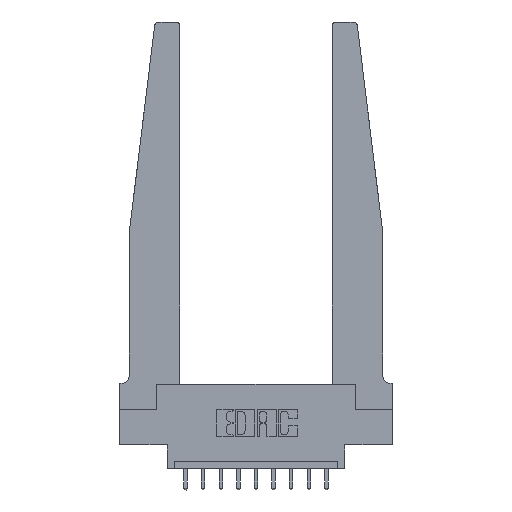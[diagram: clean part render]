
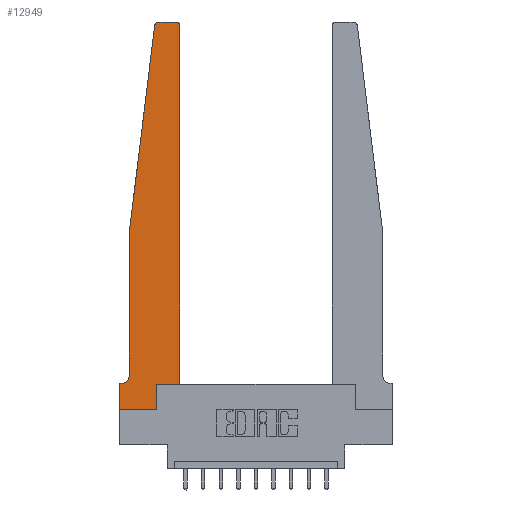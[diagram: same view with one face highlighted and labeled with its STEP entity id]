
A CAD part, top view. The second image highlights one B-rep face of the part: STEP entity #12949.
In plain terms, the highlighted planar face has unit normal (0, 0, 1).
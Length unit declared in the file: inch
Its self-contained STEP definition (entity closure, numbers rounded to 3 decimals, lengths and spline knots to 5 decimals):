
#43 = CARTESIAN_POINT ( 'NONE',  ( 0.065, 0.2375, 0.37 ) ) ;
#141 = EDGE_CURVE ( 'NONE', #6398, #14624, #8336, .T. ) ;
#646 = ORIENTED_EDGE ( 'NONE', *, *, #3364, .T. ) ;
#831 = EDGE_CURVE ( 'NONE', #3341, #6398, #3662, .T. ) ;
#875 = EDGE_CURVE ( 'NONE', #2817, #8710, #5645, .T. ) ;
#887 = LINE ( 'NONE', #10815, #14583 ) ;
#920 = DIRECTION ( 'NONE',  ( 0., -1., 0. ) ) ;
#983 = DIRECTION ( 'NONE',  ( 0., 0., 1. ) ) ;
#1242 = LINE ( 'NONE', #5475, #10400 ) ;
#1786 = DIRECTION ( 'NONE',  ( -0.122, -0.992, 0. ) ) ;
#2125 = VERTEX_POINT ( 'NONE', #9649 ) ;
#2160 = CARTESIAN_POINT ( 'NONE',  ( 0.425, 0.18, 0.37 ) ) ;
#2197 = VERTEX_POINT ( 'NONE', #4325 ) ;
#2322 = DIRECTION ( 'NONE',  ( -1., 0., 0. ) ) ;
#2430 = CARTESIAN_POINT ( 'NONE',  ( 0., 0.1875, 0.37 ) ) ;
#2730 = AXIS2_PLACEMENT_3D ( 'NONE', #3219, #983, #9914 ) ;
#2782 = CARTESIAN_POINT ( 'NONE',  ( 0.395, 2.75, 0.37 ) ) ;
#2817 = VERTEX_POINT ( 'NONE', #5413 ) ;
#3219 = CARTESIAN_POINT ( 'NONE',  ( 0.395, 2.72, 0.37 ) ) ;
#3260 = CARTESIAN_POINT ( 'NONE',  ( 0.065, 1.25, 0.37 ) ) ;
#3332 = VECTOR ( 'NONE', #11493, 39.37008 ) ;
#3341 = VERTEX_POINT ( 'NONE', #3260 ) ;
#3364 = EDGE_CURVE ( 'NONE', #8710, #3982, #12868, .T. ) ;
#3376 = ORIENTED_EDGE ( 'NONE', *, *, #875, .T. ) ;
#3406 = ORIENTED_EDGE ( 'NONE', *, *, #7383, .T. ) ;
#3469 = DIRECTION ( 'NONE',  ( 0., 1., 0. ) ) ;
#3493 = CARTESIAN_POINT ( 'NONE',  ( 0.2605, 0.18, 0.37 ) ) ;
#3662 = LINE ( 'NONE', #11194, #6195 ) ;
#3982 = VERTEX_POINT ( 'NONE', #4528 ) ;
#4040 = AXIS2_PLACEMENT_3D ( 'NONE', #13748, #14932, #2322 ) ;
#4051 = EDGE_CURVE ( 'NONE', #7455, #9309, #7421, .T. ) ;
#4325 = CARTESIAN_POINT ( 'NONE',  ( 0.425, 0.18, 0.37 ) ) ;
#4417 = PLANE ( 'NONE',  #6446 ) ;
#4528 = CARTESIAN_POINT ( 'NONE',  ( 0.27653, 2.75, 0.37 ) ) ;
#4872 = CARTESIAN_POINT ( 'NONE',  ( 0., 0., 0.37 ) ) ;
#4905 = DIRECTION ( 'NONE',  ( 1., 0., 0. ) ) ;
#5065 = LINE ( 'NONE', #2160, #12078 ) ;
#5413 = CARTESIAN_POINT ( 'NONE',  ( 0.425, 2.72, 0.37 ) ) ;
#5475 = CARTESIAN_POINT ( 'NONE',  ( 0., 0., 0.37 ) ) ;
#5494 = DIRECTION ( 'NONE',  ( -1., 0., 0. ) ) ;
#5553 = CARTESIAN_POINT ( 'NONE',  ( 0.425, 0.18, 0.37 ) ) ;
#5638 = ORIENTED_EDGE ( 'NONE', *, *, #4051, .T. ) ;
#5645 = CIRCLE ( 'NONE', #2730, 0.03 ) ;
#5825 = EDGE_CURVE ( 'NONE', #2197, #2817, #5065, .T. ) ;
#5964 = CIRCLE ( 'NONE', #11143, 0.03 ) ;
#6195 = VECTOR ( 'NONE', #13544, 39.37008 ) ;
#6284 = LINE ( 'NONE', #7845, #9150 ) ;
#6398 = VERTEX_POINT ( 'NONE', #43 ) ;
#6446 = AXIS2_PLACEMENT_3D ( 'NONE', #10159, #14784, #12630 ) ;
#6701 = DIRECTION ( 'NONE',  ( 1., 0., 0. ) ) ;
#6815 = CARTESIAN_POINT ( 'NONE',  ( 0.24675, 2.72367, 0.37 ) ) ;
#6888 = ORIENTED_EDGE ( 'NONE', *, *, #12749, .T. ) ;
#7381 = FACE_OUTER_BOUND ( 'NONE', #9390, .T. ) ;
#7383 = EDGE_CURVE ( 'NONE', #10900, #7455, #1242, .T. ) ;
#7421 = LINE ( 'NONE', #14076, #9969 ) ;
#7455 = VERTEX_POINT ( 'NONE', #4872 ) ;
#7765 = ORIENTED_EDGE ( 'NONE', *, *, #14174, .T. ) ;
#7845 = CARTESIAN_POINT ( 'NONE',  ( 0.065, 0.1875, 0.37 ) ) ;
#8004 = VERTEX_POINT ( 'NONE', #6815 ) ;
#8017 = CARTESIAN_POINT ( 'NONE',  ( 0.25, 2.75, 0.37 ) ) ;
#8221 = ORIENTED_EDGE ( 'NONE', *, *, #12568, .T. ) ;
#8263 = EDGE_CURVE ( 'NONE', #8004, #3341, #887, .T. ) ;
#8293 = ORIENTED_EDGE ( 'NONE', *, *, #141, .T. ) ;
#8336 = CIRCLE ( 'NONE', #4040, 0.05 ) ;
#8350 = CARTESIAN_POINT ( 'NONE',  ( 0.2605, 0., 0.37 ) ) ;
#8477 = VECTOR ( 'NONE', #10570, 39.37008 ) ;
#8492 = VECTOR ( 'NONE', #6701, 39.37008 ) ;
#8710 = VERTEX_POINT ( 'NONE', #2782 ) ;
#9150 = VECTOR ( 'NONE', #5494, 39.37008 ) ;
#9309 = VERTEX_POINT ( 'NONE', #8350 ) ;
#9390 = EDGE_LOOP ( 'NONE', ( #646, #6888, #13216, #11828, #8293, #7765, #3406, #5638, #8221, #12224, #14920, #3376 ) ) ;
#9649 = CARTESIAN_POINT ( 'NONE',  ( 0.2605, 0.18, 0.37 ) ) ;
#9914 = DIRECTION ( 'NONE',  ( 1., 0., 0. ) ) ;
#9969 = VECTOR ( 'NONE', #4905, 39.37008 ) ;
#10159 = CARTESIAN_POINT ( 'NONE',  ( 0., 0.1875, 0.37 ) ) ;
#10400 = VECTOR ( 'NONE', #920, 39.37008 ) ;
#10570 = DIRECTION ( 'NONE',  ( 0., 1., 0. ) ) ;
#10815 = CARTESIAN_POINT ( 'NONE',  ( 0.065, 1.25, 0.37 ) ) ;
#10900 = VERTEX_POINT ( 'NONE', #2430 ) ;
#11131 = CARTESIAN_POINT ( 'NONE',  ( 0.015, 0.1875, 0.37 ) ) ;
#11143 = AXIS2_PLACEMENT_3D ( 'NONE', #13149, #14283, #13202 ) ;
#11194 = CARTESIAN_POINT ( 'NONE',  ( 0.065, 1.25, 0.37 ) ) ;
#11493 = DIRECTION ( 'NONE',  ( -1., 0., 0. ) ) ;
#11828 = ORIENTED_EDGE ( 'NONE', *, *, #831, .T. ) ;
#11907 = LINE ( 'NONE', #5553, #8492 ) ;
#12078 = VECTOR ( 'NONE', #3469, 39.37008 ) ;
#12224 = ORIENTED_EDGE ( 'NONE', *, *, #12349, .T. ) ;
#12349 = EDGE_CURVE ( 'NONE', #2125, #2197, #11907, .T. ) ;
#12568 = EDGE_CURVE ( 'NONE', #9309, #2125, #12618, .T. ) ;
#12618 = LINE ( 'NONE', #3493, #8477 ) ;
#12630 = DIRECTION ( 'NONE',  ( 1., 0., 0. ) ) ;
#12749 = EDGE_CURVE ( 'NONE', #3982, #8004, #5964, .T. ) ;
#12868 = LINE ( 'NONE', #8017, #3332 ) ;
#12949 = ADVANCED_FACE ( 'NONE', ( #7381 ), #4417, .T. ) ;
#13149 = CARTESIAN_POINT ( 'NONE',  ( 0.27653, 2.72, 0.37 ) ) ;
#13202 = DIRECTION ( 'NONE',  ( 1., 0., 0. ) ) ;
#13216 = ORIENTED_EDGE ( 'NONE', *, *, #8263, .T. ) ;
#13544 = DIRECTION ( 'NONE',  ( 0., -1., 0. ) ) ;
#13748 = CARTESIAN_POINT ( 'NONE',  ( 0.015, 0.2375, 0.37 ) ) ;
#14076 = CARTESIAN_POINT ( 'NONE',  ( 0., 0., 0.37 ) ) ;
#14174 = EDGE_CURVE ( 'NONE', #14624, #10900, #6284, .T. ) ;
#14283 = DIRECTION ( 'NONE',  ( 0., 0., 1. ) ) ;
#14583 = VECTOR ( 'NONE', #1786, 39.37008 ) ;
#14624 = VERTEX_POINT ( 'NONE', #11131 ) ;
#14784 = DIRECTION ( 'NONE',  ( 0., 0., 1. ) ) ;
#14920 = ORIENTED_EDGE ( 'NONE', *, *, #5825, .T. ) ;
#14932 = DIRECTION ( 'NONE',  ( 0., 0., -1. ) ) ;
